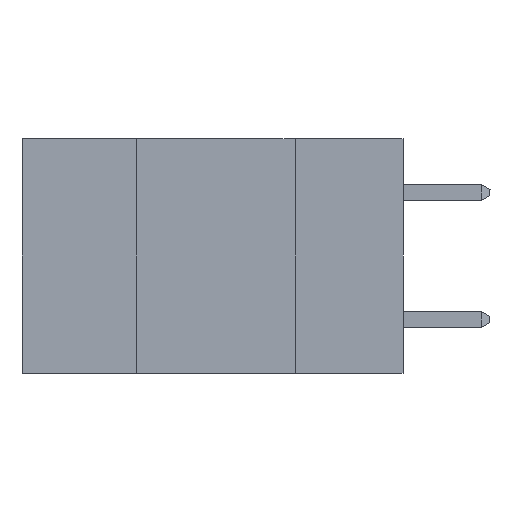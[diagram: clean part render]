
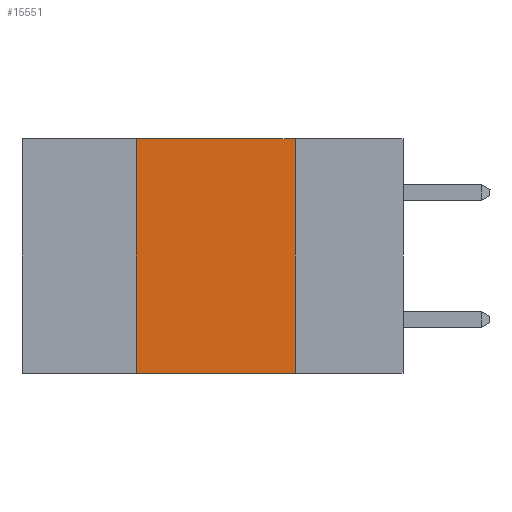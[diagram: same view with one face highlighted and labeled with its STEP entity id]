
A CAD part, left-side view. The second image highlights one B-rep face of the part: STEP entity #15551.
In plain terms, the highlighted planar face has unit normal (-1, 0, 0).
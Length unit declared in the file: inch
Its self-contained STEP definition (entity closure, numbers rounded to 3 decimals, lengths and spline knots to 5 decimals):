
#196 = LINE ( 'NONE', #19225, #22550 ) ;
#361 = CARTESIAN_POINT ( 'NONE',  ( 0., 0.6, -0.37 ) ) ;
#1292 = DIRECTION ( 'NONE',  ( 0., 0., 1. ) ) ;
#2501 = EDGE_CURVE ( 'NONE', #13469, #12413, #26867, .T. ) ;
#4398 = EDGE_CURVE ( 'NONE', #10450, #19503, #14190, .T. ) ;
#4460 = CARTESIAN_POINT ( 'NONE',  ( 0., 0.17, -0.37 ) ) ;
#4534 = CARTESIAN_POINT ( 'NONE',  ( 0., 0.6, 0. ) ) ;
#4885 = ORIENTED_EDGE ( 'NONE', *, *, #18368, .F. ) ;
#4944 = ORIENTED_EDGE ( 'NONE', *, *, #4398, .T. ) ;
#6400 = CARTESIAN_POINT ( 'NONE',  ( 0., 0.17, 0. ) ) ;
#6832 = PLANE ( 'NONE',  #17815 ) ;
#7569 = DIRECTION ( 'NONE',  ( 0., 0., -1. ) ) ;
#8001 = ORIENTED_EDGE ( 'NONE', *, *, #13119, .F. ) ;
#10450 = VERTEX_POINT ( 'NONE', #22634 ) ;
#12413 = VERTEX_POINT ( 'NONE', #6400 ) ;
#12921 = CARTESIAN_POINT ( 'NONE',  ( 0., 0.6, 0. ) ) ;
#13119 = EDGE_CURVE ( 'NONE', #12413, #19503, #196, .T. ) ;
#13329 = VECTOR ( 'NONE', #1292, 39.37008 ) ;
#13469 = VERTEX_POINT ( 'NONE', #26204 ) ;
#13996 = VECTOR ( 'NONE', #26444, 39.37008 ) ;
#14190 = LINE ( 'NONE', #361, #13996 ) ;
#15551 = ADVANCED_FACE ( 'NONE', ( #27827 ), #6832, .F. ) ;
#17815 = AXIS2_PLACEMENT_3D ( 'NONE', #4534, #23235, #21097 ) ;
#17834 = VECTOR ( 'NONE', #24872, 39.37008 ) ;
#18368 = EDGE_CURVE ( 'NONE', #10450, #13469, #19866, .T. ) ;
#19225 = CARTESIAN_POINT ( 'NONE',  ( 0., 0.17, 0. ) ) ;
#19503 = VERTEX_POINT ( 'NONE', #4460 ) ;
#19866 = LINE ( 'NONE', #24762, #13329 ) ;
#21097 = DIRECTION ( 'NONE',  ( 0., 0., -1. ) ) ;
#22550 = VECTOR ( 'NONE', #7569, 39.37008 ) ;
#22634 = CARTESIAN_POINT ( 'NONE',  ( 0., 0.42, -0.37 ) ) ;
#23235 = DIRECTION ( 'NONE',  ( 1., 0., 0. ) ) ;
#23770 = EDGE_LOOP ( 'NONE', ( #8001, #25913, #4885, #4944 ) ) ;
#24762 = CARTESIAN_POINT ( 'NONE',  ( 0., 0.42, 0. ) ) ;
#24872 = DIRECTION ( 'NONE',  ( 0., -1., 0. ) ) ;
#25913 = ORIENTED_EDGE ( 'NONE', *, *, #2501, .F. ) ;
#26204 = CARTESIAN_POINT ( 'NONE',  ( 0., 0.42, 0. ) ) ;
#26444 = DIRECTION ( 'NONE',  ( 0., -1., 0. ) ) ;
#26867 = LINE ( 'NONE', #12921, #17834 ) ;
#27827 = FACE_OUTER_BOUND ( 'NONE', #23770, .T. ) ;
